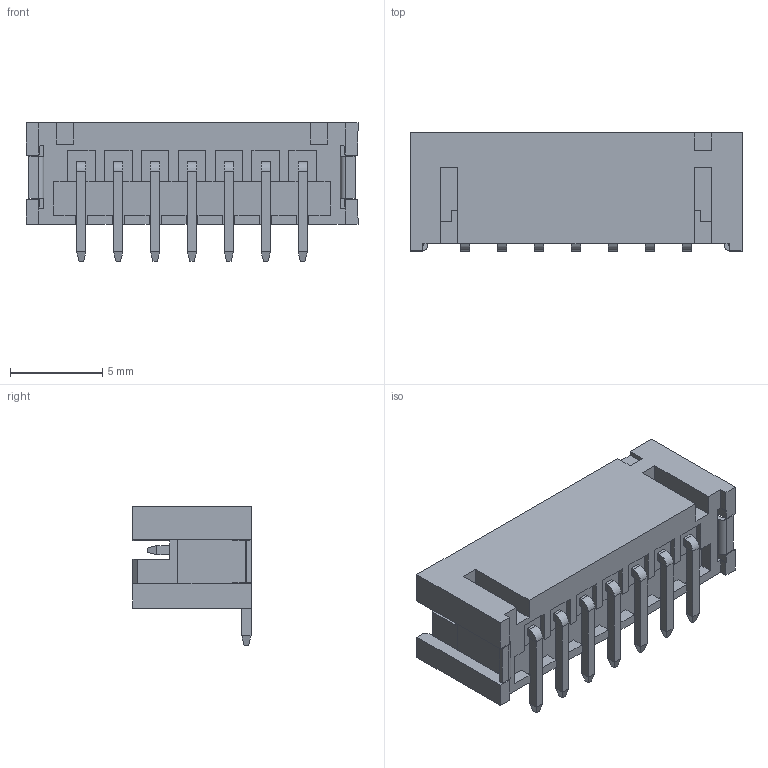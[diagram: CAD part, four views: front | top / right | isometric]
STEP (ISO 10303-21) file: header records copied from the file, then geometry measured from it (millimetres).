
FILE_DESCRIPTION (( 'STEP AP203' ), '1' );
FILE_NAME ('140-507-417-011.STEP', '2020-03-31T20:03:35', ( '' ), ( '' ), 'SwSTEP 2.0', 'SolidWorks 2016', '' );
FILE_SCHEMA (( 'CONFIG_CONTROL_DESIGN' ));
Length unit declared in the file: millimetre
Products named in the file (4): 140-507-417-011; V SMT Pad; V SMT Contact; V SMT Housing_507
Assembly tree (10 placements, depth 2):
  140-507-417-011
    V SMT Housing_507
    V SMT Contact  x7
    V SMT Pad  x2
Bounding box: 18 x 6.4 x 7.5 mm (x, y, z)
Volume: 274.1 mm3; surface area: 984.9 mm2
Topology: 10 solids, 10 shells, 366 faces, 928 edges, 578 vertices
Faces by surface type: plane 348, cylinder 18
Entity records: 7666 total; most frequent: CARTESIAN_POINT 1271, ORIENTED_EDGE 1256, DIRECTION 1102, EDGE_CURVE 628, VECTOR 620, LINE 620, VERTEX_POINT 410, AXIS2_PLACEMENT_3D 241
